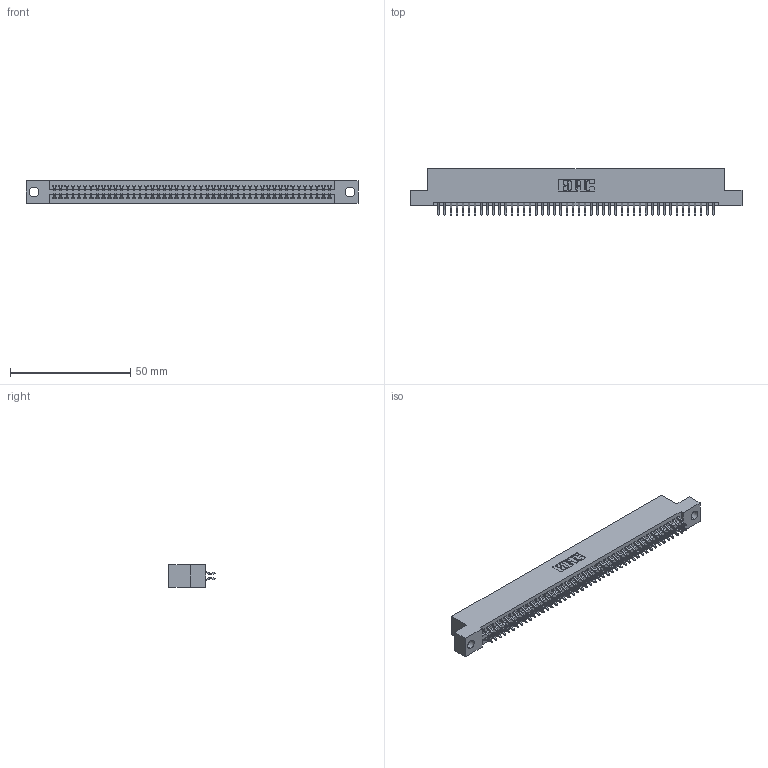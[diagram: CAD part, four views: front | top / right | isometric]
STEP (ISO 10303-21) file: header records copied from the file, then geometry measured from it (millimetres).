
FILE_DESCRIPTION (( 'STEP AP203' ), '1' );
FILE_NAME ('345-092-556-204.STEP', '2021-05-20T15:51:06', ( '' ), ( '' ), 'SwSTEP 2.0', 'SolidWorks 2020', '' );
FILE_SCHEMA (( 'CONFIG_CONTROL_DESIGN' ));
Length unit declared in the file: inch
Products named in the file (3): 345-292-001_556 Tail; 345 Part_Flush Mounting Lugs - 0.156 Dia-TI; 345-092-556-204
Assembly tree (93 placements, depth 2):
  345-092-556-204
    345 Part_Flush Mounting Lugs - 0.156 Dia-TI
    345-292-001_556 Tail  x92
Bounding box: 138.05 x 19.24 x 9.4 mm (x, y, z)
Volume: 13337.8 mm3; surface area: 19564 mm2
Topology: 93 solids, 93 shells, 5292 faces, 15741 edges, 10370 vertices
Faces by surface type: plane 3498, cylinder 1794
Entity records: 36193 total; most frequent: CARTESIAN_POINT 6082, ORIENTED_EDGE 6002, DIRECTION 5345, EDGE_CURVE 3001, VECTOR 2677, LINE 2677, VERTEX_POINT 1998, AXIS2_PLACEMENT_3D 1334
